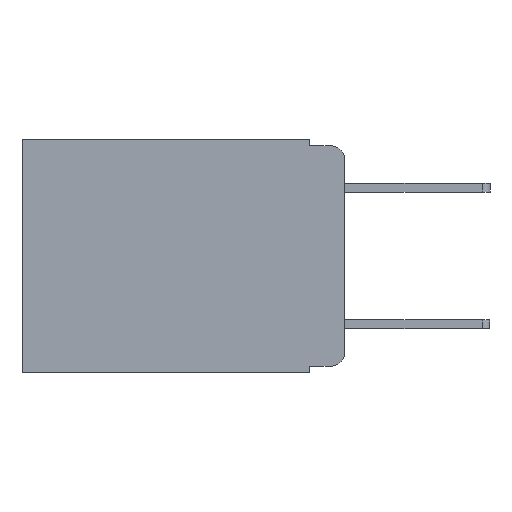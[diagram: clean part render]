
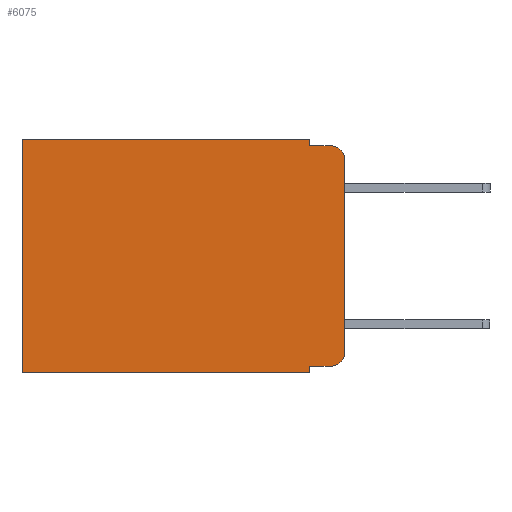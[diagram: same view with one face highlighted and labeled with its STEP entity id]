
A CAD part, left-side view. The second image highlights one B-rep face of the part: STEP entity #6075.
In plain terms, the highlighted planar face has unit normal (-1, 0, 0).
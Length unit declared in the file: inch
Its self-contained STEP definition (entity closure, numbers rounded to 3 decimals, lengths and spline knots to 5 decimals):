
#17 = VERTEX_POINT ( 'NONE', #7000 ) ;
#34 = VECTOR ( 'NONE', #8132, 39.37008 ) ;
#309 = DIRECTION ( 'NONE',  ( 1., 0., 0. ) ) ;
#947 = CARTESIAN_POINT ( 'NONE',  ( 0.298, 0.473, 0. ) ) ;
#1018 = EDGE_CURVE ( 'NONE', #1261, #4193, #2783, .T. ) ;
#1107 = DIRECTION ( 'NONE',  ( 0., 0., -1. ) ) ;
#1261 = VERTEX_POINT ( 'NONE', #2328 ) ;
#1313 = FACE_OUTER_BOUND ( 'NONE', #5385, .T. ) ;
#1501 = LINE ( 'NONE', #8981, #6384 ) ;
#1597 = CIRCLE ( 'NONE', #5775, 0.02 ) ;
#1653 = DIRECTION ( 'NONE',  ( 0., -1., 0. ) ) ;
#1722 = EDGE_CURVE ( 'NONE', #9694, #10490, #1501, .T. ) ;
#1949 = CARTESIAN_POINT ( 'NONE',  ( 0.298, 0.051, 0. ) ) ;
#2010 = VERTEX_POINT ( 'NONE', #5510 ) ;
#2096 = LINE ( 'NONE', #4937, #11637 ) ;
#2328 = CARTESIAN_POINT ( 'NONE',  ( 0.298, 0.051, -0.333 ) ) ;
#2471 = VECTOR ( 'NONE', #11914, 39.37008 ) ;
#2477 = DIRECTION ( 'NONE',  ( -1., 0., 0. ) ) ;
#2544 = CARTESIAN_POINT ( 'NONE',  ( 0.298, 0.051, 0. ) ) ;
#2573 = ORIENTED_EDGE ( 'NONE', *, *, #9895, .T. ) ;
#2579 = CARTESIAN_POINT ( 'NONE',  ( 0.298, 0.051, -0.01 ) ) ;
#2621 = ORIENTED_EDGE ( 'NONE', *, *, #7621, .T. ) ;
#2627 = CARTESIAN_POINT ( 'NONE',  ( 0.298, 0.051, -0.343 ) ) ;
#2691 = VECTOR ( 'NONE', #1653, 39.37008 ) ;
#2783 = LINE ( 'NONE', #1949, #2471 ) ;
#3040 = VERTEX_POINT ( 'NONE', #3962 ) ;
#3042 = LINE ( 'NONE', #4365, #34 ) ;
#3082 = EDGE_CURVE ( 'NONE', #1261, #4879, #2096, .T. ) ;
#3117 = AXIS2_PLACEMENT_3D ( 'NONE', #9781, #309, #7160 ) ;
#3528 = ORIENTED_EDGE ( 'NONE', *, *, #3977, .F. ) ;
#3956 = CARTESIAN_POINT ( 'NONE',  ( 0.298, 0., -0.03 ) ) ;
#3962 = CARTESIAN_POINT ( 'NONE',  ( 0.298, 0.051, 0. ) ) ;
#3977 = EDGE_CURVE ( 'NONE', #12041, #2010, #7754, .T. ) ;
#4077 = ORIENTED_EDGE ( 'NONE', *, *, #11967, .T. ) ;
#4142 = EDGE_CURVE ( 'NONE', #3040, #12041, #6018, .T. ) ;
#4193 = VERTEX_POINT ( 'NONE', #2627 ) ;
#4296 = ORIENTED_EDGE ( 'NONE', *, *, #6154, .F. ) ;
#4365 = CARTESIAN_POINT ( 'NONE',  ( 0.298, 0., -0.343 ) ) ;
#4370 = CARTESIAN_POINT ( 'NONE',  ( 0.298, 0.02, -0.03 ) ) ;
#4561 = ORIENTED_EDGE ( 'NONE', *, *, #7243, .T. ) ;
#4625 = VERTEX_POINT ( 'NONE', #947 ) ;
#4818 = ORIENTED_EDGE ( 'NONE', *, *, #4142, .F. ) ;
#4879 = VERTEX_POINT ( 'NONE', #6490 ) ;
#4937 = CARTESIAN_POINT ( 'NONE',  ( 0.298, 0.051, -0.333 ) ) ;
#5078 = ORIENTED_EDGE ( 'NONE', *, *, #3082, .T. ) ;
#5227 = ORIENTED_EDGE ( 'NONE', *, *, #1018, .F. ) ;
#5380 = DIRECTION ( 'NONE',  ( 0., 0., -1. ) ) ;
#5385 = EDGE_LOOP ( 'NONE', ( #6697, #4561, #3528, #4818, #4077, #2621, #4296, #5227, #5078, #2573 ) ) ;
#5510 = CARTESIAN_POINT ( 'NONE',  ( 0.298, 0.02, -0.01 ) ) ;
#5726 = VECTOR ( 'NONE', #11132, 39.37008 ) ;
#5775 = AXIS2_PLACEMENT_3D ( 'NONE', #4370, #10807, #5380 ) ;
#6018 = LINE ( 'NONE', #2544, #5726 ) ;
#6075 = ADVANCED_FACE ( 'NONE', ( #1313 ), #11552, .F. ) ;
#6154 = EDGE_CURVE ( 'NONE', #4193, #17, #3042, .T. ) ;
#6384 = VECTOR ( 'NONE', #6872, 39.37008 ) ;
#6490 = CARTESIAN_POINT ( 'NONE',  ( 0.298, 0.02, -0.333 ) ) ;
#6697 = ORIENTED_EDGE ( 'NONE', *, *, #1722, .F. ) ;
#6768 = VECTOR ( 'NONE', #1107, 39.37008 ) ;
#6813 = AXIS2_PLACEMENT_3D ( 'NONE', #8158, #2477, #9092 ) ;
#6872 = DIRECTION ( 'NONE',  ( 0., 0., -1. ) ) ;
#6952 = CARTESIAN_POINT ( 'NONE',  ( 0.298, 0.473, 0. ) ) ;
#7000 = CARTESIAN_POINT ( 'NONE',  ( 0.298, 0.473, -0.343 ) ) ;
#7150 = LINE ( 'NONE', #8008, #11834 ) ;
#7160 = DIRECTION ( 'NONE',  ( 0., 0., -1. ) ) ;
#7243 = EDGE_CURVE ( 'NONE', #9694, #2010, #1597, .T. ) ;
#7621 = EDGE_CURVE ( 'NONE', #4625, #17, #11214, .T. ) ;
#7754 = LINE ( 'NONE', #2579, #2691 ) ;
#8008 = CARTESIAN_POINT ( 'NONE',  ( 0.298, 0., 0. ) ) ;
#8087 = CARTESIAN_POINT ( 'NONE',  ( 0.298, 0.051, -0.01 ) ) ;
#8132 = DIRECTION ( 'NONE',  ( 0., 1., 0. ) ) ;
#8158 = CARTESIAN_POINT ( 'NONE',  ( 0.298, 0.02, -0.313 ) ) ;
#8981 = CARTESIAN_POINT ( 'NONE',  ( 0.298, 0., 0. ) ) ;
#9092 = DIRECTION ( 'NONE',  ( 0., 0., -1. ) ) ;
#9694 = VERTEX_POINT ( 'NONE', #3956 ) ;
#9781 = CARTESIAN_POINT ( 'NONE',  ( 0.298, 0., 0. ) ) ;
#9895 = EDGE_CURVE ( 'NONE', #4879, #10490, #11226, .T. ) ;
#10490 = VERTEX_POINT ( 'NONE', #11647 ) ;
#10670 = DIRECTION ( 'NONE',  ( 0., 1., 0. ) ) ;
#10807 = DIRECTION ( 'NONE',  ( -1., 0., 0. ) ) ;
#10976 = DIRECTION ( 'NONE',  ( 0., -1., 0. ) ) ;
#11132 = DIRECTION ( 'NONE',  ( 0., 0., -1. ) ) ;
#11214 = LINE ( 'NONE', #6952, #6768 ) ;
#11226 = CIRCLE ( 'NONE', #6813, 0.02 ) ;
#11552 = PLANE ( 'NONE',  #3117 ) ;
#11637 = VECTOR ( 'NONE', #10976, 39.37008 ) ;
#11647 = CARTESIAN_POINT ( 'NONE',  ( 0.298, 0., -0.313 ) ) ;
#11834 = VECTOR ( 'NONE', #10670, 39.37008 ) ;
#11914 = DIRECTION ( 'NONE',  ( 0., 0., -1. ) ) ;
#11967 = EDGE_CURVE ( 'NONE', #3040, #4625, #7150, .T. ) ;
#12041 = VERTEX_POINT ( 'NONE', #8087 ) ;
